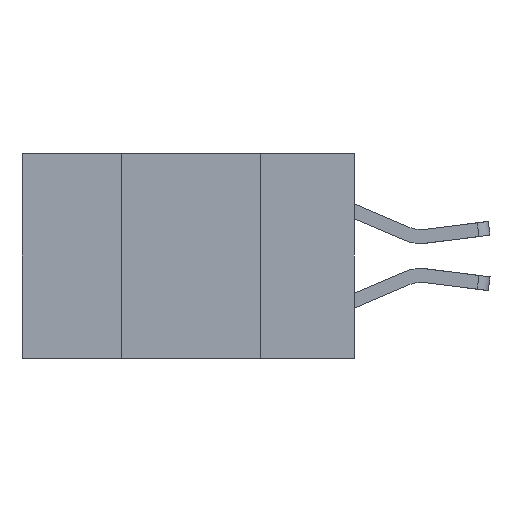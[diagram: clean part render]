
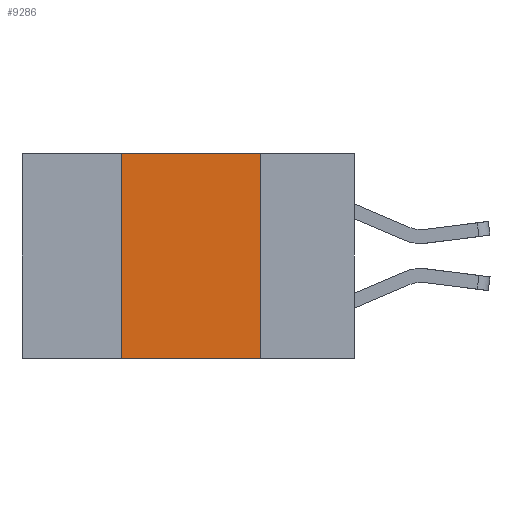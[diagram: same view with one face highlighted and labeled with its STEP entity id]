
A CAD part, left-side view. The second image highlights one B-rep face of the part: STEP entity #9286.
In plain terms, the highlighted planar face has unit normal (-1, 0, 0).
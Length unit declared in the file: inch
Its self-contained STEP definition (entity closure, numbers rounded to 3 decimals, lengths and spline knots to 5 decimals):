
#955 = VECTOR ( 'NONE', #7502, 39.37008 ) ;
#1169 = VERTEX_POINT ( 'NONE', #6635 ) ;
#1225 = VECTOR ( 'NONE', #4016, 39.37008 ) ;
#1510 = LINE ( 'NONE', #7681, #1225 ) ;
#2292 = CARTESIAN_POINT ( 'NONE',  ( 0., 0.42, 0. ) ) ;
#2821 = EDGE_CURVE ( 'NONE', #5483, #8671, #5920, .T. ) ;
#3047 = CARTESIAN_POINT ( 'NONE',  ( 0., 0.6, 0. ) ) ;
#3180 = AXIS2_PLACEMENT_3D ( 'NONE', #5808, #5063, #5094 ) ;
#3696 = VECTOR ( 'NONE', #3896, 39.37008 ) ;
#3880 = EDGE_CURVE ( 'NONE', #8671, #9815, #9211, .T. ) ;
#3896 = DIRECTION ( 'NONE',  ( 0., 0., 1. ) ) ;
#4016 = DIRECTION ( 'NONE',  ( 0., 0., -1. ) ) ;
#4028 = CARTESIAN_POINT ( 'NONE',  ( 0., 0.6, -0.37 ) ) ;
#4076 = EDGE_CURVE ( 'NONE', #5483, #1169, #9324, .T. ) ;
#4358 = PLANE ( 'NONE',  #3180 ) ;
#4897 = EDGE_CURVE ( 'NONE', #9815, #1169, #1510, .T. ) ;
#5063 = DIRECTION ( 'NONE',  ( 1., 0., 0. ) ) ;
#5094 = DIRECTION ( 'NONE',  ( 0., 0., -1. ) ) ;
#5483 = VERTEX_POINT ( 'NONE', #7352 ) ;
#5808 = CARTESIAN_POINT ( 'NONE',  ( 0., 0.6, 0. ) ) ;
#5920 = LINE ( 'NONE', #9758, #3696 ) ;
#5937 = EDGE_LOOP ( 'NONE', ( #9222, #7284, #9197, #7167 ) ) ;
#6635 = CARTESIAN_POINT ( 'NONE',  ( 0., 0.17, -0.37 ) ) ;
#6925 = CARTESIAN_POINT ( 'NONE',  ( 0., 0.17, 0. ) ) ;
#7167 = ORIENTED_EDGE ( 'NONE', *, *, #4076, .T. ) ;
#7284 = ORIENTED_EDGE ( 'NONE', *, *, #3880, .F. ) ;
#7352 = CARTESIAN_POINT ( 'NONE',  ( 0., 0.42, -0.37 ) ) ;
#7386 = VECTOR ( 'NONE', #9882, 39.37008 ) ;
#7502 = DIRECTION ( 'NONE',  ( 0., -1., 0. ) ) ;
#7681 = CARTESIAN_POINT ( 'NONE',  ( 0., 0.17, -0.37 ) ) ;
#8671 = VERTEX_POINT ( 'NONE', #2292 ) ;
#9197 = ORIENTED_EDGE ( 'NONE', *, *, #2821, .F. ) ;
#9211 = LINE ( 'NONE', #3047, #955 ) ;
#9222 = ORIENTED_EDGE ( 'NONE', *, *, #4897, .F. ) ;
#9286 = ADVANCED_FACE ( 'NONE', ( #9361 ), #4358, .F. ) ;
#9324 = LINE ( 'NONE', #4028, #7386 ) ;
#9361 = FACE_OUTER_BOUND ( 'NONE', #5937, .T. ) ;
#9758 = CARTESIAN_POINT ( 'NONE',  ( 0., 0.42, -0.37 ) ) ;
#9815 = VERTEX_POINT ( 'NONE', #6925 ) ;
#9882 = DIRECTION ( 'NONE',  ( 0., -1., 0. ) ) ;
